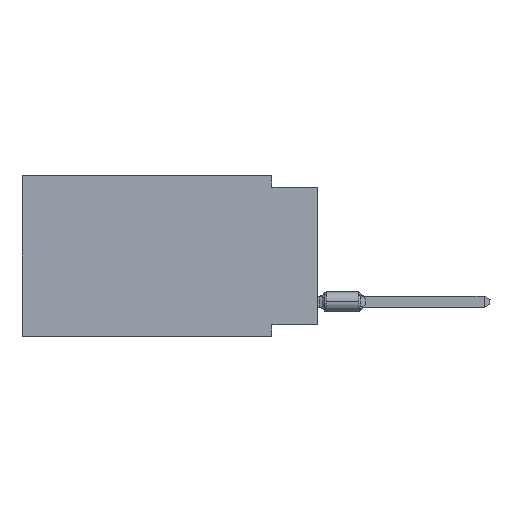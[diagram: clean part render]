
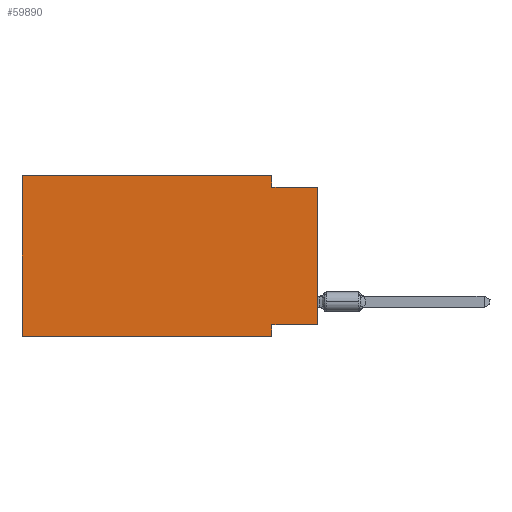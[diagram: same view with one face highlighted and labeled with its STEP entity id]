
A CAD part, left-side view. The second image highlights one B-rep face of the part: STEP entity #59890.
In plain terms, the highlighted planar face has unit normal (-1, 0, 0).
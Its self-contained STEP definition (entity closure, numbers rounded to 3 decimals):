
#897 = CARTESIAN_POINT ( 'NONE',  ( 0., 0., -8.255 ) ) ;
#2918 = VECTOR ( 'NONE', #29319, 1000. ) ;
#6454 = VECTOR ( 'NONE', #10033, 1000. ) ;
#7108 = DIRECTION ( 'NONE',  ( 0., 0., -1. ) ) ;
#7381 = CARTESIAN_POINT ( 'NONE',  ( 0., 2.54, -8.89 ) ) ;
#8478 = CARTESIAN_POINT ( 'NONE',  ( 0., 0., -8.255 ) ) ;
#8695 = LINE ( 'NONE', #23862, #62241 ) ;
#10033 = DIRECTION ( 'NONE',  ( 0., 0., 1. ) ) ;
#10572 = VECTOR ( 'NONE', #22876, 1000. ) ;
#10968 = ORIENTED_EDGE ( 'NONE', *, *, #44431, .F. ) ;
#12488 = VERTEX_POINT ( 'NONE', #21684 ) ;
#13001 = EDGE_CURVE ( 'NONE', #54314, #12488, #48711, .T. ) ;
#13088 = DIRECTION ( 'NONE',  ( 0., -1., 0. ) ) ;
#13980 = CARTESIAN_POINT ( 'NONE',  ( 0., 2.54, 0. ) ) ;
#14320 = VECTOR ( 'NONE', #42876, 1000. ) ;
#14416 = CARTESIAN_POINT ( 'NONE',  ( 0., 2.54, -8.89 ) ) ;
#15095 = LINE ( 'NONE', #25528, #6454 ) ;
#15678 = VERTEX_POINT ( 'NONE', #61875 ) ;
#16542 = DIRECTION ( 'NONE',  ( 1., 0., 0. ) ) ;
#16823 = VERTEX_POINT ( 'NONE', #21355 ) ;
#17050 = LINE ( 'NONE', #52590, #14320 ) ;
#20440 = ORIENTED_EDGE ( 'NONE', *, *, #47031, .T. ) ;
#20616 = ORIENTED_EDGE ( 'NONE', *, *, #49354, .F. ) ;
#21054 = EDGE_CURVE ( 'NONE', #54314, #58549, #64178, .T. ) ;
#21355 = CARTESIAN_POINT ( 'NONE',  ( 0., 2.54, -0.635 ) ) ;
#21684 = CARTESIAN_POINT ( 'NONE',  ( 0., 0., -0.635 ) ) ;
#22876 = DIRECTION ( 'NONE',  ( 0., 0., -1. ) ) ;
#23862 = CARTESIAN_POINT ( 'NONE',  ( 0., 16.383, 0. ) ) ;
#25528 = CARTESIAN_POINT ( 'NONE',  ( 0., 16.383, 0. ) ) ;
#26199 = ORIENTED_EDGE ( 'NONE', *, *, #13001, .T. ) ;
#26974 = PLANE ( 'NONE',  #51959 ) ;
#28983 = VERTEX_POINT ( 'NONE', #50454 ) ;
#29319 = DIRECTION ( 'NONE',  ( 0., 1., 0. ) ) ;
#30401 = VECTOR ( 'NONE', #47655, 1000. ) ;
#32788 = EDGE_CURVE ( 'NONE', #28983, #42056, #15095, .T. ) ;
#34389 = VERTEX_POINT ( 'NONE', #14416 ) ;
#38851 = LINE ( 'NONE', #13980, #43442 ) ;
#39897 = VECTOR ( 'NONE', #48394, 1000. ) ;
#41303 = ORIENTED_EDGE ( 'NONE', *, *, #32788, .F. ) ;
#41889 = EDGE_CURVE ( 'NONE', #58549, #34389, #63100, .T. ) ;
#42056 = VERTEX_POINT ( 'NONE', #53688 ) ;
#42290 = CARTESIAN_POINT ( 'NONE',  ( 0., 16.383, -8.89 ) ) ;
#42876 = DIRECTION ( 'NONE',  ( 0., -1., 0. ) ) ;
#43442 = VECTOR ( 'NONE', #44855, 1000. ) ;
#44431 = EDGE_CURVE ( 'NONE', #42056, #15678, #8695, .T. ) ;
#44624 = ORIENTED_EDGE ( 'NONE', *, *, #21054, .F. ) ;
#44855 = DIRECTION ( 'NONE',  ( 0., 0., -1. ) ) ;
#47031 = EDGE_CURVE ( 'NONE', #28983, #34389, #57696, .T. ) ;
#47655 = DIRECTION ( 'NONE',  ( 0., -1., 0. ) ) ;
#47743 = CARTESIAN_POINT ( 'NONE',  ( 0., 16.383, 0. ) ) ;
#48069 = FACE_OUTER_BOUND ( 'NONE', #59146, .T. ) ;
#48394 = DIRECTION ( 'NONE',  ( 0., 0., 1. ) ) ;
#48711 = LINE ( 'NONE', #53080, #39897 ) ;
#49354 = EDGE_CURVE ( 'NONE', #15678, #16823, #38851, .T. ) ;
#50454 = CARTESIAN_POINT ( 'NONE',  ( 0., 16.383, -8.89 ) ) ;
#50792 = CARTESIAN_POINT ( 'NONE',  ( 0., 2.54, -8.255 ) ) ;
#51959 = AXIS2_PLACEMENT_3D ( 'NONE', #47743, #16542, #7108 ) ;
#52590 = CARTESIAN_POINT ( 'NONE',  ( 0., 0., -0.635 ) ) ;
#53080 = CARTESIAN_POINT ( 'NONE',  ( 0., 0., 0. ) ) ;
#53688 = CARTESIAN_POINT ( 'NONE',  ( 0., 16.383, 0. ) ) ;
#54314 = VERTEX_POINT ( 'NONE', #897 ) ;
#57696 = LINE ( 'NONE', #42290, #30401 ) ;
#58549 = VERTEX_POINT ( 'NONE', #50792 ) ;
#58667 = EDGE_CURVE ( 'NONE', #16823, #12488, #17050, .T. ) ;
#59146 = EDGE_LOOP ( 'NONE', ( #26199, #66307, #20616, #10968, #41303, #20440, #60330, #44624 ) ) ;
#59890 = ADVANCED_FACE ( 'NONE', ( #48069 ), #26974, .F. ) ;
#60330 = ORIENTED_EDGE ( 'NONE', *, *, #41889, .F. ) ;
#61875 = CARTESIAN_POINT ( 'NONE',  ( 0., 2.54, 0. ) ) ;
#62241 = VECTOR ( 'NONE', #13088, 1000. ) ;
#63100 = LINE ( 'NONE', #7381, #10572 ) ;
#64178 = LINE ( 'NONE', #8478, #2918 ) ;
#66307 = ORIENTED_EDGE ( 'NONE', *, *, #58667, .F. ) ;
